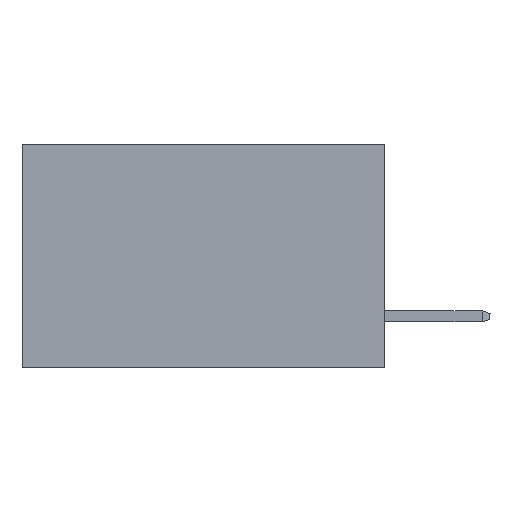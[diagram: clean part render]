
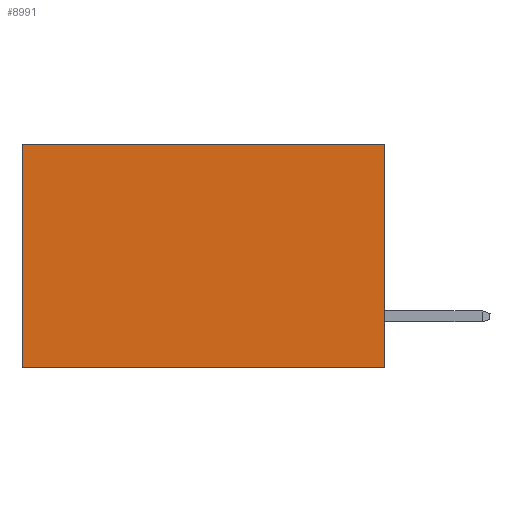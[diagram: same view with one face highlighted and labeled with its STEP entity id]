
A CAD part, left-side view. The second image highlights one B-rep face of the part: STEP entity #8991.
In plain terms, the highlighted planar face has unit normal (-1, 0, 0).
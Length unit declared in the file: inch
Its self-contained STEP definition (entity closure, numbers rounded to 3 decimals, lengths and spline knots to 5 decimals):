
#421 = VERTEX_POINT ( 'NONE', #3912 ) ;
#1008 = LINE ( 'NONE', #21254, #15529 ) ;
#1145 = DIRECTION ( 'NONE',  ( 0., 0., -1. ) ) ;
#2477 = CARTESIAN_POINT ( 'NONE',  ( 0.2615, 0., 0. ) ) ;
#2514 = EDGE_CURVE ( 'NONE', #12470, #21477, #13935, .T. ) ;
#3449 = ORIENTED_EDGE ( 'NONE', *, *, #14576, .F. ) ;
#3912 = CARTESIAN_POINT ( 'NONE',  ( 0.2615, 0.6, 0. ) ) ;
#4714 = LINE ( 'NONE', #2477, #5715 ) ;
#5310 = AXIS2_PLACEMENT_3D ( 'NONE', #7447, #15330, #24827 ) ;
#5684 = LINE ( 'NONE', #13575, #21717 ) ;
#5715 = VECTOR ( 'NONE', #24438, 39.37008 ) ;
#7209 = CARTESIAN_POINT ( 'NONE',  ( 0.2615, 0.6, -0.37 ) ) ;
#7447 = CARTESIAN_POINT ( 'NONE',  ( 0.2615, 0., -0.37 ) ) ;
#7800 = DIRECTION ( 'NONE',  ( 0., 0., -1. ) ) ;
#8789 = EDGE_CURVE ( 'NONE', #13993, #421, #4714, .T. ) ;
#8991 = ADVANCED_FACE ( 'NONE', ( #11254 ), #23716, .F. ) ;
#11123 = CARTESIAN_POINT ( 'NONE',  ( 0.2615, 0., -0.37 ) ) ;
#11254 = FACE_OUTER_BOUND ( 'NONE', #15457, .T. ) ;
#12470 = VERTEX_POINT ( 'NONE', #11123 ) ;
#13429 = DIRECTION ( 'NONE',  ( 0., 1., 0. ) ) ;
#13575 = CARTESIAN_POINT ( 'NONE',  ( 0.2615, 0., -0.37 ) ) ;
#13935 = LINE ( 'NONE', #15666, #20250 ) ;
#13993 = VERTEX_POINT ( 'NONE', #15468 ) ;
#14576 = EDGE_CURVE ( 'NONE', #13993, #12470, #5684, .T. ) ;
#15330 = DIRECTION ( 'NONE',  ( 1., 0., 0. ) ) ;
#15457 = EDGE_LOOP ( 'NONE', ( #21324, #21718, #3449, #24932 ) ) ;
#15468 = CARTESIAN_POINT ( 'NONE',  ( 0.2615, 0., 0. ) ) ;
#15529 = VECTOR ( 'NONE', #1145, 39.37008 ) ;
#15666 = CARTESIAN_POINT ( 'NONE',  ( 0.2615, 0., -0.37 ) ) ;
#20250 = VECTOR ( 'NONE', #13429, 39.37008 ) ;
#21254 = CARTESIAN_POINT ( 'NONE',  ( 0.2615, 0.6, -0.37 ) ) ;
#21324 = ORIENTED_EDGE ( 'NONE', *, *, #22969, .T. ) ;
#21477 = VERTEX_POINT ( 'NONE', #7209 ) ;
#21717 = VECTOR ( 'NONE', #7800, 39.37008 ) ;
#21718 = ORIENTED_EDGE ( 'NONE', *, *, #2514, .F. ) ;
#22969 = EDGE_CURVE ( 'NONE', #421, #21477, #1008, .T. ) ;
#23716 = PLANE ( 'NONE',  #5310 ) ;
#24438 = DIRECTION ( 'NONE',  ( 0., 1., 0. ) ) ;
#24827 = DIRECTION ( 'NONE',  ( 0., 0., -1. ) ) ;
#24932 = ORIENTED_EDGE ( 'NONE', *, *, #8789, .T. ) ;
